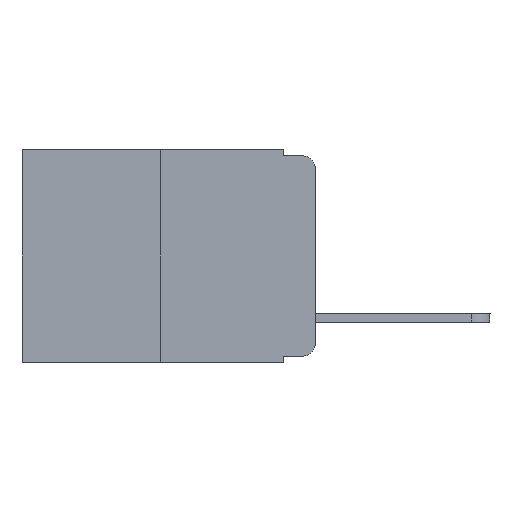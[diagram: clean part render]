
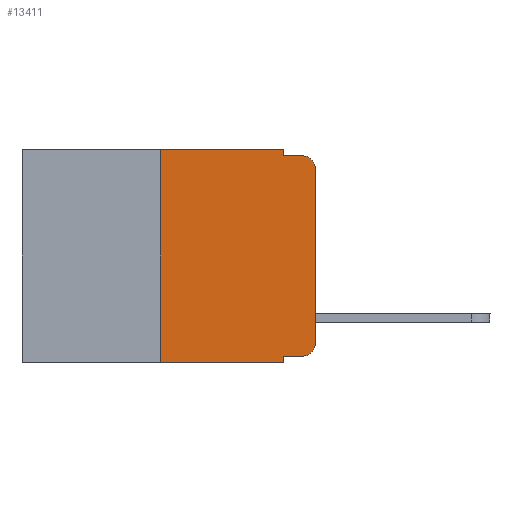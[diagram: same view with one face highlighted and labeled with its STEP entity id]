
A CAD part, left-side view. The second image highlights one B-rep face of the part: STEP entity #13411.
In plain terms, the highlighted planar face has unit normal (-1, 0, 0).
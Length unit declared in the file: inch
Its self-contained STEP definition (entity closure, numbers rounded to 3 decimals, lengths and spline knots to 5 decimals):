
#56 = ORIENTED_EDGE ( 'NONE', *, *, #4983, .T. ) ;
#493 = LINE ( 'NONE', #1633, #3318 ) ;
#619 = PLANE ( 'NONE',  #10097 ) ;
#817 = CARTESIAN_POINT ( 'NONE',  ( 0., 0.051, -0.333 ) ) ;
#863 = CARTESIAN_POINT ( 'NONE',  ( 0., 0.473, 0. ) ) ;
#893 = DIRECTION ( 'NONE',  ( 0., -1., 0. ) ) ;
#988 = EDGE_CURVE ( 'NONE', #6827, #1652, #11971, .T. ) ;
#1044 = CARTESIAN_POINT ( 'NONE',  ( 0., 0.02, -0.01 ) ) ;
#1595 = CARTESIAN_POINT ( 'NONE',  ( 0., 0.02, -0.03 ) ) ;
#1633 = CARTESIAN_POINT ( 'NONE',  ( 0., 0.051, 0. ) ) ;
#1644 = VECTOR ( 'NONE', #9348, 39.37008 ) ;
#1652 = VERTEX_POINT ( 'NONE', #11201 ) ;
#1862 = ORIENTED_EDGE ( 'NONE', *, *, #2131, .F. ) ;
#2131 = EDGE_CURVE ( 'NONE', #5725, #12655, #6899, .T. ) ;
#2197 = CARTESIAN_POINT ( 'NONE',  ( 0., 0.051, -0.333 ) ) ;
#2460 = VERTEX_POINT ( 'NONE', #10152 ) ;
#2486 = CARTESIAN_POINT ( 'NONE',  ( 0., 0.051, -0.01 ) ) ;
#3179 = CARTESIAN_POINT ( 'NONE',  ( 0., 0.25, 0. ) ) ;
#3318 = VECTOR ( 'NONE', #4310, 39.37008 ) ;
#3965 = EDGE_CURVE ( 'NONE', #1652, #2460, #6381, .T. ) ;
#4009 = EDGE_LOOP ( 'NONE', ( #56, #6459, #13668, #10770, #14413, #1862, #10202, #8170, #11592, #4521 ) ) ;
#4017 = VERTEX_POINT ( 'NONE', #14936 ) ;
#4216 = EDGE_CURVE ( 'NONE', #4527, #14274, #12989, .T. ) ;
#4310 = DIRECTION ( 'NONE',  ( 0., 0., -1. ) ) ;
#4521 = ORIENTED_EDGE ( 'NONE', *, *, #3965, .T. ) ;
#4527 = VERTEX_POINT ( 'NONE', #13981 ) ;
#4676 = DIRECTION ( 'NONE',  ( 1., 0., 0. ) ) ;
#4796 = EDGE_CURVE ( 'NONE', #12655, #4017, #16054, .T. ) ;
#4983 = EDGE_CURVE ( 'NONE', #2460, #4527, #11497, .T. ) ;
#5490 = CARTESIAN_POINT ( 'NONE',  ( 0., 0.051, -0.01 ) ) ;
#5721 = AXIS2_PLACEMENT_3D ( 'NONE', #1595, #11534, #10294 ) ;
#5725 = VERTEX_POINT ( 'NONE', #8520 ) ;
#5771 = VERTEX_POINT ( 'NONE', #2486 ) ;
#5908 = CARTESIAN_POINT ( 'NONE',  ( 0., 0.051, 0. ) ) ;
#5946 = CARTESIAN_POINT ( 'NONE',  ( 0., 0.25, 0. ) ) ;
#5975 = CARTESIAN_POINT ( 'NONE',  ( 0., 0.473, 0. ) ) ;
#6142 = LINE ( 'NONE', #5908, #11378 ) ;
#6381 = CIRCLE ( 'NONE', #12639, 0.02 ) ;
#6459 = ORIENTED_EDGE ( 'NONE', *, *, #4216, .T. ) ;
#6520 = CARTESIAN_POINT ( 'NONE',  ( 0., 0., 0. ) ) ;
#6827 = VERTEX_POINT ( 'NONE', #817 ) ;
#6899 = LINE ( 'NONE', #3179, #1644 ) ;
#7057 = DIRECTION ( 'NONE',  ( 0., 0., -1. ) ) ;
#7800 = EDGE_CURVE ( 'NONE', #5725, #14178, #8679, .T. ) ;
#7957 = VECTOR ( 'NONE', #9043, 39.37008 ) ;
#8170 = ORIENTED_EDGE ( 'NONE', *, *, #10744, .F. ) ;
#8290 = DIRECTION ( 'NONE',  ( -1., 0., 0. ) ) ;
#8520 = CARTESIAN_POINT ( 'NONE',  ( 0., 0.25, -0.343 ) ) ;
#8679 = LINE ( 'NONE', #8757, #13734 ) ;
#8757 = CARTESIAN_POINT ( 'NONE',  ( 0., 0.473, -0.343 ) ) ;
#9002 = VECTOR ( 'NONE', #12264, 39.37008 ) ;
#9043 = DIRECTION ( 'NONE',  ( 0., 0., 1. ) ) ;
#9295 = LINE ( 'NONE', #5490, #14093 ) ;
#9348 = DIRECTION ( 'NONE',  ( 0., 0., 1. ) ) ;
#9596 = VECTOR ( 'NONE', #893, 39.37008 ) ;
#10097 = AXIS2_PLACEMENT_3D ( 'NONE', #863, #4676, #13326 ) ;
#10151 = EDGE_CURVE ( 'NONE', #4017, #5771, #493, .T. ) ;
#10152 = CARTESIAN_POINT ( 'NONE',  ( 0., 0., -0.313 ) ) ;
#10202 = ORIENTED_EDGE ( 'NONE', *, *, #7800, .T. ) ;
#10294 = DIRECTION ( 'NONE',  ( 0., 0., -1. ) ) ;
#10744 = EDGE_CURVE ( 'NONE', #6827, #14178, #6142, .T. ) ;
#10770 = ORIENTED_EDGE ( 'NONE', *, *, #10151, .F. ) ;
#10870 = DIRECTION ( 'NONE',  ( 0., 0., -1. ) ) ;
#11201 = CARTESIAN_POINT ( 'NONE',  ( 0., 0.02, -0.333 ) ) ;
#11378 = VECTOR ( 'NONE', #10870, 39.37008 ) ;
#11497 = LINE ( 'NONE', #6520, #7957 ) ;
#11534 = DIRECTION ( 'NONE',  ( -1., 0., 0. ) ) ;
#11592 = ORIENTED_EDGE ( 'NONE', *, *, #988, .T. ) ;
#11765 = FACE_OUTER_BOUND ( 'NONE', #4009, .T. ) ;
#11971 = LINE ( 'NONE', #2197, #9596 ) ;
#12264 = DIRECTION ( 'NONE',  ( 0., -1., 0. ) ) ;
#12639 = AXIS2_PLACEMENT_3D ( 'NONE', #14521, #8290, #7057 ) ;
#12655 = VERTEX_POINT ( 'NONE', #5946 ) ;
#12989 = CIRCLE ( 'NONE', #5721, 0.02 ) ;
#13326 = DIRECTION ( 'NONE',  ( 0., 0., -1. ) ) ;
#13411 = ADVANCED_FACE ( 'NONE', ( #11765 ), #619, .F. ) ;
#13668 = ORIENTED_EDGE ( 'NONE', *, *, #15010, .F. ) ;
#13734 = VECTOR ( 'NONE', #14993, 39.37008 ) ;
#13981 = CARTESIAN_POINT ( 'NONE',  ( 0., 0., -0.03 ) ) ;
#14093 = VECTOR ( 'NONE', #15633, 39.37008 ) ;
#14178 = VERTEX_POINT ( 'NONE', #15841 ) ;
#14274 = VERTEX_POINT ( 'NONE', #1044 ) ;
#14413 = ORIENTED_EDGE ( 'NONE', *, *, #4796, .F. ) ;
#14521 = CARTESIAN_POINT ( 'NONE',  ( 0., 0.02, -0.313 ) ) ;
#14936 = CARTESIAN_POINT ( 'NONE',  ( 0., 0.051, 0. ) ) ;
#14993 = DIRECTION ( 'NONE',  ( 0., -1., 0. ) ) ;
#15010 = EDGE_CURVE ( 'NONE', #5771, #14274, #9295, .T. ) ;
#15633 = DIRECTION ( 'NONE',  ( 0., -1., 0. ) ) ;
#15841 = CARTESIAN_POINT ( 'NONE',  ( 0., 0.051, -0.343 ) ) ;
#16054 = LINE ( 'NONE', #5975, #9002 ) ;
